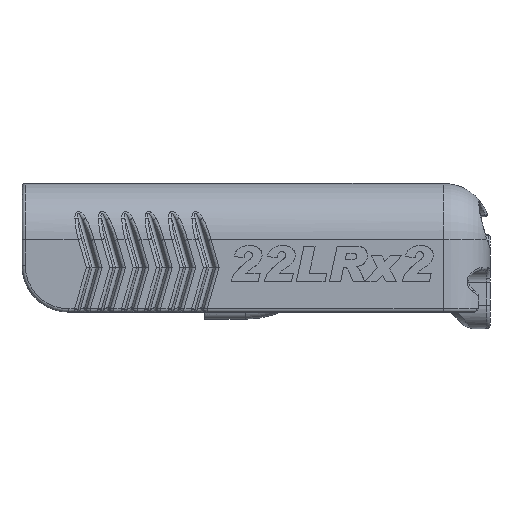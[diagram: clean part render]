
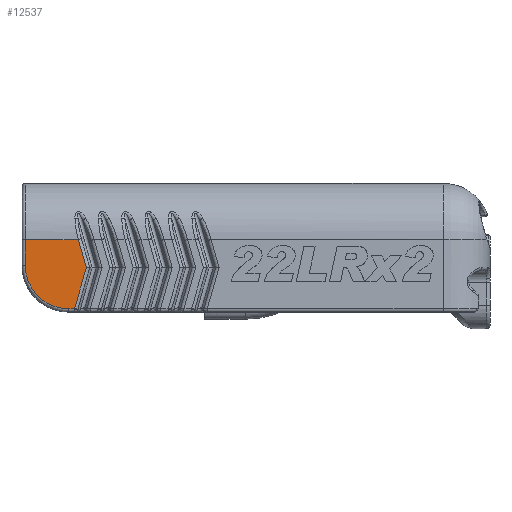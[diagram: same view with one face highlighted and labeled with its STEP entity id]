
A CAD part, front view. The second image highlights one B-rep face of the part: STEP entity #12537.
In plain terms, the highlighted planar face has unit normal (0, -1, 0).
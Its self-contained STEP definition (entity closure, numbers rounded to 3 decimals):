
#33 = CYLINDRICAL_SURFACE('',#34,12.);
#34 = AXIS2_PLACEMENT_3D('',#35,#36,#37);
#35 = CARTESIAN_POINT('',(0.,-3.,-3.));
#36 = DIRECTION('',(1.,0.,0.));
#37 = DIRECTION('',(0.,-1.,0.));
#3822 = VERTEX_POINT('',#3823);
#3823 = CARTESIAN_POINT('',(12.024,-15.,-3.));
#3879 = EDGE_CURVE('',#3880,#3822,#3882,.T.);
#3880 = VERTEX_POINT('',#3881);
#3881 = CARTESIAN_POINT('',(0.7,-15.,-3.));
#3882 = SURFACE_CURVE('',#3883,(#3887,#3894),.PCURVE_S1.);
#3883 = LINE('',#3884,#3885);
#3884 = CARTESIAN_POINT('',(0.,-15.,-3.));
#3885 = VECTOR('',#3886,1.);
#3886 = DIRECTION('',(1.,0.,0.));
#3887 = PCURVE('',#33,#3888);
#3888 = DEFINITIONAL_REPRESENTATION('',(#3889),#3893);
#3889 = LINE('',#3890,#3891);
#3890 = CARTESIAN_POINT('',(-0.,0.));
#3891 = VECTOR('',#3892,1.);
#3892 = DIRECTION('',(-0.,1.));
#3893 = ( GEOMETRIC_REPRESENTATION_CONTEXT(2) 
PARAMETRIC_REPRESENTATION_CONTEXT() REPRESENTATION_CONTEXT('2D SPACE',''
  ) );
#3894 = PCURVE('',#3895,#3900);
#3895 = PLANE('',#3896);
#3896 = AXIS2_PLACEMENT_3D('',#3897,#3898,#3899);
#3897 = CARTESIAN_POINT('',(0.,-15.,-18.5));
#3898 = DIRECTION('',(0.,1.,0.));
#3899 = DIRECTION('',(0.,0.,1.));
#3900 = DEFINITIONAL_REPRESENTATION('',(#3901),#3905);
#3901 = LINE('',#3902,#3903);
#3902 = CARTESIAN_POINT('',(15.5,0.));
#3903 = VECTOR('',#3904,1.);
#3904 = DIRECTION('',(0.,1.));
#3905 = ( GEOMETRIC_REPRESENTATION_CONTEXT(2) 
PARAMETRIC_REPRESENTATION_CONTEXT() REPRESENTATION_CONTEXT('2D SPACE',''
  ) );
#12520 = CYLINDRICAL_SURFACE('',#12521,0.8);
#12521 = AXIS2_PLACEMENT_3D('',#12522,#12523,#12524);
#12522 = CARTESIAN_POINT('',(12.061,-14.2,-3.127));
#12523 = DIRECTION('',(0.276,0.,-0.961));
#12524 = DIRECTION('',(0.,-1.,0.));
#12537 = ADVANCED_FACE('',(#12538),#3895,.F.);
#12538 = FACE_BOUND('',#12539,.F.);
#12539 = EDGE_LOOP('',(#12540,#12570,#12599,#12625,#12626,#12649,#12677)
  );
#12540 = ORIENTED_EDGE('',*,*,#12541,.T.);
#12541 = EDGE_CURVE('',#12542,#12544,#12546,.T.);
#12542 = VERTEX_POINT('',#12543);
#12543 = CARTESIAN_POINT('',(11.226,-15.,-17.8));
#12544 = VERTEX_POINT('',#12545);
#12545 = CARTESIAN_POINT('',(10.,-15.,-17.8));
#12546 = SURFACE_CURVE('',#12547,(#12551,#12558),.PCURVE_S1.);
#12547 = LINE('',#12548,#12549);
#12548 = CARTESIAN_POINT('',(90.,-15.,-17.8));
#12549 = VECTOR('',#12550,1.);
#12550 = DIRECTION('',(-1.,-0.,-0.));
#12551 = PCURVE('',#3895,#12552);
#12552 = DEFINITIONAL_REPRESENTATION('',(#12553),#12557);
#12553 = LINE('',#12554,#12555);
#12554 = CARTESIAN_POINT('',(0.7,90.));
#12555 = VECTOR('',#12556,1.);
#12556 = DIRECTION('',(-0.,-1.));
#12557 = ( GEOMETRIC_REPRESENTATION_CONTEXT(2) 
PARAMETRIC_REPRESENTATION_CONTEXT() REPRESENTATION_CONTEXT('2D SPACE',''
  ) );
#12558 = PCURVE('',#12559,#12564);
#12559 = CYLINDRICAL_SURFACE('',#12560,0.7);
#12560 = AXIS2_PLACEMENT_3D('',#12561,#12562,#12563);
#12561 = CARTESIAN_POINT('',(90.,-14.3,-17.8));
#12562 = DIRECTION('',(-1.,-0.,-0.));
#12563 = DIRECTION('',(0.,-1.,0.));
#12564 = DEFINITIONAL_REPRESENTATION('',(#12565),#12569);
#12565 = LINE('',#12566,#12567);
#12566 = CARTESIAN_POINT('',(-0.,0.));
#12567 = VECTOR('',#12568,1.);
#12568 = DIRECTION('',(-0.,1.));
#12569 = ( GEOMETRIC_REPRESENTATION_CONTEXT(2) 
PARAMETRIC_REPRESENTATION_CONTEXT() REPRESENTATION_CONTEXT('2D SPACE',''
  ) );
#12570 = ORIENTED_EDGE('',*,*,#12571,.T.);
#12571 = EDGE_CURVE('',#12544,#12572,#12574,.T.);
#12572 = VERTEX_POINT('',#12573);
#12573 = CARTESIAN_POINT('',(0.7,-15.,-8.5));
#12574 = SURFACE_CURVE('',#12575,(#12580,#12587),.PCURVE_S1.);
#12575 = CIRCLE('',#12576,9.3);
#12576 = AXIS2_PLACEMENT_3D('',#12577,#12578,#12579);
#12577 = CARTESIAN_POINT('',(10.,-15.,-8.5));
#12578 = DIRECTION('',(0.,1.,0.));
#12579 = DIRECTION('',(0.,0.,-1.));
#12580 = PCURVE('',#3895,#12581);
#12581 = DEFINITIONAL_REPRESENTATION('',(#12582),#12586);
#12582 = CIRCLE('',#12583,9.3);
#12583 = AXIS2_PLACEMENT_2D('',#12584,#12585);
#12584 = CARTESIAN_POINT('',(10.,10.));
#12585 = DIRECTION('',(-1.,0.));
#12586 = ( GEOMETRIC_REPRESENTATION_CONTEXT(2) 
PARAMETRIC_REPRESENTATION_CONTEXT() REPRESENTATION_CONTEXT('2D SPACE',''
  ) );
#12587 = PCURVE('',#12588,#12593);
#12588 = TOROIDAL_SURFACE('',#12589,9.3,0.7);
#12589 = AXIS2_PLACEMENT_3D('',#12590,#12591,#12592);
#12590 = CARTESIAN_POINT('',(10.,-14.3,-8.5));
#12591 = DIRECTION('',(0.,1.,0.));
#12592 = DIRECTION('',(0.,0.,-1.));
#12593 = DEFINITIONAL_REPRESENTATION('',(#12594),#12598);
#12594 = LINE('',#12595,#12596);
#12595 = CARTESIAN_POINT('',(0.,4.712));
#12596 = VECTOR('',#12597,1.);
#12597 = DIRECTION('',(1.,0.));
#12598 = ( GEOMETRIC_REPRESENTATION_CONTEXT(2) 
PARAMETRIC_REPRESENTATION_CONTEXT() REPRESENTATION_CONTEXT('2D SPACE',''
  ) );
#12599 = ORIENTED_EDGE('',*,*,#12600,.T.);
#12600 = EDGE_CURVE('',#12572,#3880,#12601,.T.);
#12601 = SURFACE_CURVE('',#12602,(#12606,#12613),.PCURVE_S1.);
#12602 = LINE('',#12603,#12604);
#12603 = CARTESIAN_POINT('',(0.7,-15.,-8.5));
#12604 = VECTOR('',#12605,1.);
#12605 = DIRECTION('',(0.,0.,1.));
#12606 = PCURVE('',#3895,#12607);
#12607 = DEFINITIONAL_REPRESENTATION('',(#12608),#12612);
#12608 = LINE('',#12609,#12610);
#12609 = CARTESIAN_POINT('',(10.,0.7));
#12610 = VECTOR('',#12611,1.);
#12611 = DIRECTION('',(1.,0.));
#12612 = ( GEOMETRIC_REPRESENTATION_CONTEXT(2) 
PARAMETRIC_REPRESENTATION_CONTEXT() REPRESENTATION_CONTEXT('2D SPACE',''
  ) );
#12613 = PCURVE('',#12614,#12619);
#12614 = CYLINDRICAL_SURFACE('',#12615,0.7);
#12615 = AXIS2_PLACEMENT_3D('',#12616,#12617,#12618);
#12616 = CARTESIAN_POINT('',(0.7,-14.3,-8.5));
#12617 = DIRECTION('',(0.,0.,1.));
#12618 = DIRECTION('',(0.,-1.,0.));
#12619 = DEFINITIONAL_REPRESENTATION('',(#12620),#12624);
#12620 = LINE('',#12621,#12622);
#12621 = CARTESIAN_POINT('',(-0.,0.));
#12622 = VECTOR('',#12623,1.);
#12623 = DIRECTION('',(-0.,1.));
#12624 = ( GEOMETRIC_REPRESENTATION_CONTEXT(2) 
PARAMETRIC_REPRESENTATION_CONTEXT() REPRESENTATION_CONTEXT('2D SPACE',''
  ) );
#12625 = ORIENTED_EDGE('',*,*,#3879,.T.);
#12626 = ORIENTED_EDGE('',*,*,#12627,.T.);
#12627 = EDGE_CURVE('',#3822,#12628,#12630,.T.);
#12628 = VERTEX_POINT('',#12629);
#12629 = CARTESIAN_POINT('',(13.745,-15.,-9.));
#12630 = SURFACE_CURVE('',#12631,(#12635,#12642),.PCURVE_S1.);
#12631 = LINE('',#12632,#12633);
#12632 = CARTESIAN_POINT('',(12.061,-15.,-3.127));
#12633 = VECTOR('',#12634,1.);
#12634 = DIRECTION('',(0.276,0.,-0.961));
#12635 = PCURVE('',#3895,#12636);
#12636 = DEFINITIONAL_REPRESENTATION('',(#12637),#12641);
#12637 = LINE('',#12638,#12639);
#12638 = CARTESIAN_POINT('',(15.373,12.061));
#12639 = VECTOR('',#12640,1.);
#12640 = DIRECTION('',(-0.961,0.276));
#12641 = ( GEOMETRIC_REPRESENTATION_CONTEXT(2) 
PARAMETRIC_REPRESENTATION_CONTEXT() REPRESENTATION_CONTEXT('2D SPACE',''
  ) );
#12642 = PCURVE('',#12520,#12643);
#12643 = DEFINITIONAL_REPRESENTATION('',(#12644),#12648);
#12644 = LINE('',#12645,#12646);
#12645 = CARTESIAN_POINT('',(-0.,0.));
#12646 = VECTOR('',#12647,1.);
#12647 = DIRECTION('',(-0.,1.));
#12648 = ( GEOMETRIC_REPRESENTATION_CONTEXT(2) 
PARAMETRIC_REPRESENTATION_CONTEXT() REPRESENTATION_CONTEXT('2D SPACE',''
  ) );
#12649 = ORIENTED_EDGE('',*,*,#12650,.F.);
#12650 = EDGE_CURVE('',#12651,#12628,#12653,.T.);
#12651 = VERTEX_POINT('',#12652);
#12652 = CARTESIAN_POINT('',(11.258,-15.,-17.673));
#12653 = SURFACE_CURVE('',#12654,(#12658,#12665),.PCURVE_S1.);
#12654 = LINE('',#12655,#12656);
#12655 = CARTESIAN_POINT('',(11.258,-15.,-17.673));
#12656 = VECTOR('',#12657,1.);
#12657 = DIRECTION('',(0.276,0.,0.961));
#12658 = PCURVE('',#3895,#12659);
#12659 = DEFINITIONAL_REPRESENTATION('',(#12660),#12664);
#12660 = LINE('',#12661,#12662);
#12661 = CARTESIAN_POINT('',(0.827,11.258));
#12662 = VECTOR('',#12663,1.);
#12663 = DIRECTION('',(0.961,0.276));
#12664 = ( GEOMETRIC_REPRESENTATION_CONTEXT(2) 
PARAMETRIC_REPRESENTATION_CONTEXT() REPRESENTATION_CONTEXT('2D SPACE',''
  ) );
#12665 = PCURVE('',#12666,#12671);
#12666 = CYLINDRICAL_SURFACE('',#12667,0.8);
#12667 = AXIS2_PLACEMENT_3D('',#12668,#12669,#12670);
#12668 = CARTESIAN_POINT('',(11.258,-14.2,-17.673));
#12669 = DIRECTION('',(0.276,0.,0.961));
#12670 = DIRECTION('',(0.,-1.,0.));
#12671 = DEFINITIONAL_REPRESENTATION('',(#12672),#12676);
#12672 = LINE('',#12673,#12674);
#12673 = CARTESIAN_POINT('',(0.,0.));
#12674 = VECTOR('',#12675,1.);
#12675 = DIRECTION('',(0.,1.));
#12676 = ( GEOMETRIC_REPRESENTATION_CONTEXT(2) 
PARAMETRIC_REPRESENTATION_CONTEXT() REPRESENTATION_CONTEXT('2D SPACE',''
  ) );
#12677 = ORIENTED_EDGE('',*,*,#12678,.F.);
#12678 = EDGE_CURVE('',#12542,#12651,#12679,.T.);
#12679 = SURFACE_CURVE('',#12680,(#12685,#12693),.PCURVE_S1.);
#12680 = ( BOUNDED_CURVE() B_SPLINE_CURVE(3,(#12681,#12682,#12683,#12684
),.UNSPECIFIED.,.F.,.F.) B_SPLINE_CURVE_WITH_KNOTS((4,4),(
13.842,13.94),.PIECEWISE_BEZIER_KNOTS.) CURVE() 
GEOMETRIC_REPRESENTATION_ITEM() RATIONAL_B_SPLINE_CURVE((1.,1.,1.,1.)) 
REPRESENTATION_ITEM('') );
#12681 = CARTESIAN_POINT('',(11.226,-15.,-17.8));
#12682 = CARTESIAN_POINT('',(11.235,-15.,-17.757));
#12683 = CARTESIAN_POINT('',(11.246,-15.,-17.715));
#12684 = CARTESIAN_POINT('',(11.258,-15.,-17.673));
#12685 = PCURVE('',#3895,#12686);
#12686 = DEFINITIONAL_REPRESENTATION('',(#12687),#12692);
#12687 = B_SPLINE_CURVE_WITH_KNOTS('',3,(#12688,#12689,#12690,#12691),
  .UNSPECIFIED.,.F.,.F.,(4,4),(13.842,13.94),
  .PIECEWISE_BEZIER_KNOTS.);
#12688 = CARTESIAN_POINT('',(0.7,11.226));
#12689 = CARTESIAN_POINT('',(0.743,11.235));
#12690 = CARTESIAN_POINT('',(0.785,11.246));
#12691 = CARTESIAN_POINT('',(0.827,11.258));
#12692 = ( GEOMETRIC_REPRESENTATION_CONTEXT(2) 
PARAMETRIC_REPRESENTATION_CONTEXT() REPRESENTATION_CONTEXT('2D SPACE',''
  ) );
#12693 = PCURVE('',#12694,#12707);
#12694 = ( BOUNDED_SURFACE() B_SPLINE_SURFACE(2,3,(
    (#12695,#12696,#12697,#12698)
    ,(#12699,#12700,#12701,#12702)
    ,(#12703,#12704,#12705,#12706
)),.UNSPECIFIED.,.F.,.F.,.F.) B_SPLINE_SURFACE_WITH_KNOTS((3,3),(4,4),(
    0.,0.098),(13.842,13.94),
.PIECEWISE_BEZIER_KNOTS.) GEOMETRIC_REPRESENTATION_ITEM() 
RATIONAL_B_SPLINE_SURFACE((
    (1.,1.,1.,1.)
    ,(0.867,0.866,0.866,0.866)
,(1.,1.,1.,1.))) REPRESENTATION_ITEM('') SURFACE() );
#12695 = CARTESIAN_POINT('',(11.226,-15.,-17.8));
#12696 = CARTESIAN_POINT('',(11.235,-15.,-17.757));
#12697 = CARTESIAN_POINT('',(11.246,-15.,-17.715));
#12698 = CARTESIAN_POINT('',(11.258,-15.,-17.673));
#12699 = CARTESIAN_POINT('',(11.675,-15.,-17.893));
#12700 = CARTESIAN_POINT('',(11.684,-15.,-17.862));
#12701 = CARTESIAN_POINT('',(11.693,-15.,-17.831));
#12702 = CARTESIAN_POINT('',(11.702,-15.,-17.8));
#12703 = CARTESIAN_POINT('',(11.913,-14.607,
    -17.889));
#12704 = CARTESIAN_POINT('',(11.918,-14.602,
    -17.881));
#12705 = CARTESIAN_POINT('',(11.921,-14.6,-17.873));
#12706 = CARTESIAN_POINT('',(11.924,-14.6,-17.864));
#12707 = DEFINITIONAL_REPRESENTATION('',(#12708),#12712);
#12708 = LINE('',#12709,#12710);
#12709 = CARTESIAN_POINT('',(0.,0.));
#12710 = VECTOR('',#12711,1.);
#12711 = DIRECTION('',(0.,1.));
#12712 = ( GEOMETRIC_REPRESENTATION_CONTEXT(2) 
PARAMETRIC_REPRESENTATION_CONTEXT() REPRESENTATION_CONTEXT('2D SPACE',''
  ) );
